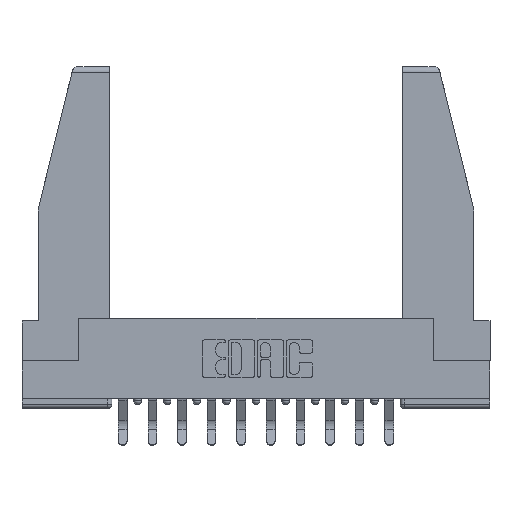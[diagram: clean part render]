
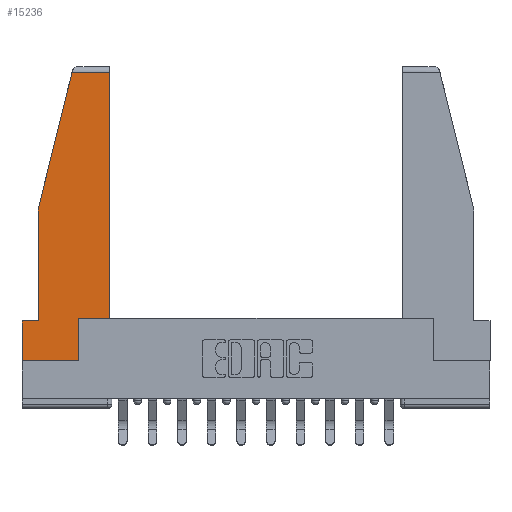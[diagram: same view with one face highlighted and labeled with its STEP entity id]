
A CAD part, top view. The second image highlights one B-rep face of the part: STEP entity #15236.
In plain terms, the highlighted planar face has unit normal (0, 0, 1).
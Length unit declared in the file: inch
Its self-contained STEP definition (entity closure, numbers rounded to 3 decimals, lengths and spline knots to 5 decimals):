
#5 = EDGE_CURVE ( 'NONE', #15086, #2855, #11032, .T. ) ;
#369 = LINE ( 'NONE', #2797, #9836 ) ;
#1672 = CARTESIAN_POINT ( 'NONE',  ( 0., 0.21, 0. ) ) ;
#1780 = DIRECTION ( 'NONE',  ( -1., 0., 0. ) ) ;
#1796 = VERTEX_POINT ( 'NONE', #14291 ) ;
#1830 = EDGE_LOOP ( 'NONE', ( #7287, #4741, #14758, #6312, #3966, #5749, #7761, #8469, #12510 ) ) ;
#2246 = CARTESIAN_POINT ( 'NONE',  ( 0.297, 0., 0. ) ) ;
#2334 = VECTOR ( 'NONE', #3683, 39.37008 ) ;
#2590 = CARTESIAN_POINT ( 'NONE',  ( 0., 0., 0. ) ) ;
#2641 = VECTOR ( 'NONE', #9715, 39.37008 ) ;
#2797 = CARTESIAN_POINT ( 'NONE',  ( 0.297, 0., 0. ) ) ;
#2804 = DIRECTION ( 'NONE',  ( 0., 0., 1. ) ) ;
#2854 = DIRECTION ( 'NONE',  ( 1., 0., 0. ) ) ;
#2855 = VERTEX_POINT ( 'NONE', #2246 ) ;
#3161 = CARTESIAN_POINT ( 'NONE',  ( 0.461, 1.52, 0. ) ) ;
#3273 = EDGE_CURVE ( 'NONE', #3718, #1796, #11835, .T. ) ;
#3510 = VECTOR ( 'NONE', #12122, 39.37008 ) ;
#3683 = DIRECTION ( 'NONE',  ( -1., 0., 0. ) ) ;
#3718 = VERTEX_POINT ( 'NONE', #10244 ) ;
#3784 = EDGE_CURVE ( 'NONE', #11024, #6812, #4551, .T. ) ;
#3813 = LINE ( 'NONE', #9623, #2334 ) ;
#3966 = ORIENTED_EDGE ( 'NONE', *, *, #3273, .T. ) ;
#4099 = CARTESIAN_POINT ( 'NONE',  ( 0., 0., 0. ) ) ;
#4340 = CARTESIAN_POINT ( 'NONE',  ( 0.2636, 1.52, 0. ) ) ;
#4551 = LINE ( 'NONE', #5278, #12757 ) ;
#4741 = ORIENTED_EDGE ( 'NONE', *, *, #13007, .T. ) ;
#5032 = VERTEX_POINT ( 'NONE', #3161 ) ;
#5082 = PLANE ( 'NONE',  #7135 ) ;
#5177 = EDGE_CURVE ( 'NONE', #11028, #12932, #7126, .T. ) ;
#5278 = CARTESIAN_POINT ( 'NONE',  ( 0.297, 0.223, 0. ) ) ;
#5636 = VECTOR ( 'NONE', #13625, 39.37008 ) ;
#5738 = EDGE_CURVE ( 'NONE', #6812, #5032, #11264, .T. ) ;
#5749 = ORIENTED_EDGE ( 'NONE', *, *, #9218, .T. ) ;
#6312 = ORIENTED_EDGE ( 'NONE', *, *, #6777, .T. ) ;
#6385 = DIRECTION ( 'NONE',  ( 0., -1., 0. ) ) ;
#6459 = LINE ( 'NONE', #1672, #13915 ) ;
#6755 = VECTOR ( 'NONE', #8828, 39.37008 ) ;
#6777 = EDGE_CURVE ( 'NONE', #12932, #3718, #9669, .T. ) ;
#6812 = VERTEX_POINT ( 'NONE', #13277 ) ;
#7126 = LINE ( 'NONE', #13567, #6755 ) ;
#7135 = AXIS2_PLACEMENT_3D ( 'NONE', #4099, #2804, #2854 ) ;
#7287 = ORIENTED_EDGE ( 'NONE', *, *, #5738, .T. ) ;
#7448 = EDGE_CURVE ( 'NONE', #2855, #11024, #369, .T. ) ;
#7527 = CARTESIAN_POINT ( 'NONE',  ( 0.086, 0.8, 0. ) ) ;
#7761 = ORIENTED_EDGE ( 'NONE', *, *, #5, .T. ) ;
#8463 = CARTESIAN_POINT ( 'NONE',  ( 0.086, 0.8, 0. ) ) ;
#8469 = ORIENTED_EDGE ( 'NONE', *, *, #7448, .T. ) ;
#8828 = DIRECTION ( 'NONE',  ( -0.239, -0.971, 0. ) ) ;
#8873 = VECTOR ( 'NONE', #1780, 39.37008 ) ;
#9218 = EDGE_CURVE ( 'NONE', #1796, #15086, #6459, .T. ) ;
#9623 = CARTESIAN_POINT ( 'NONE',  ( 0., 1.52, 0. ) ) ;
#9669 = LINE ( 'NONE', #7527, #3510 ) ;
#9715 = DIRECTION ( 'NONE',  ( 1., 0., 0. ) ) ;
#9745 = DIRECTION ( 'NONE',  ( 0., 1., 0. ) ) ;
#9836 = VECTOR ( 'NONE', #9745, 39.37008 ) ;
#10244 = CARTESIAN_POINT ( 'NONE',  ( 0.086, 0.21, 0. ) ) ;
#10877 = CARTESIAN_POINT ( 'NONE',  ( 0., 0., 0. ) ) ;
#11024 = VERTEX_POINT ( 'NONE', #14913 ) ;
#11028 = VERTEX_POINT ( 'NONE', #4340 ) ;
#11032 = LINE ( 'NONE', #10877, #2641 ) ;
#11259 = CARTESIAN_POINT ( 'NONE',  ( 0., 0.21, 0. ) ) ;
#11264 = LINE ( 'NONE', #14866, #5636 ) ;
#11835 = LINE ( 'NONE', #11259, #8873 ) ;
#12122 = DIRECTION ( 'NONE',  ( 0., -1., 0. ) ) ;
#12510 = ORIENTED_EDGE ( 'NONE', *, *, #3784, .T. ) ;
#12757 = VECTOR ( 'NONE', #14916, 39.37008 ) ;
#12932 = VERTEX_POINT ( 'NONE', #8463 ) ;
#13007 = EDGE_CURVE ( 'NONE', #5032, #11028, #3813, .T. ) ;
#13277 = CARTESIAN_POINT ( 'NONE',  ( 0.461, 0.223, 0. ) ) ;
#13567 = CARTESIAN_POINT ( 'NONE',  ( 0.271, 1.55, 0. ) ) ;
#13625 = DIRECTION ( 'NONE',  ( 0., 1., 0. ) ) ;
#13915 = VECTOR ( 'NONE', #6385, 39.37008 ) ;
#14291 = CARTESIAN_POINT ( 'NONE',  ( 0., 0.21, 0. ) ) ;
#14747 = FACE_OUTER_BOUND ( 'NONE', #1830, .T. ) ;
#14758 = ORIENTED_EDGE ( 'NONE', *, *, #5177, .T. ) ;
#14866 = CARTESIAN_POINT ( 'NONE',  ( 0.461, 0.223, 0. ) ) ;
#14913 = CARTESIAN_POINT ( 'NONE',  ( 0.297, 0.223, 0. ) ) ;
#14916 = DIRECTION ( 'NONE',  ( 1., 0., 0. ) ) ;
#15086 = VERTEX_POINT ( 'NONE', #2590 ) ;
#15236 = ADVANCED_FACE ( 'NONE', ( #14747 ), #5082, .T. ) ;
